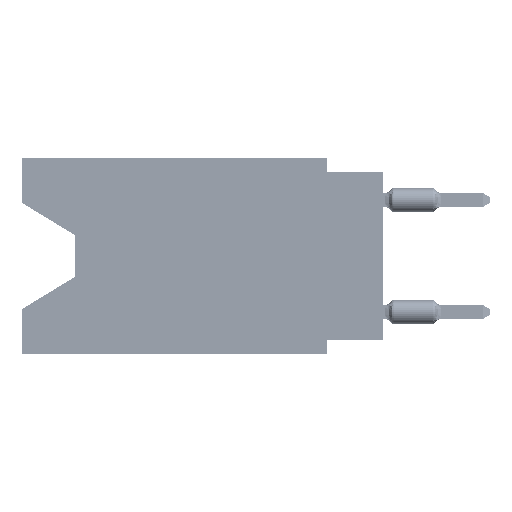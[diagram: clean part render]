
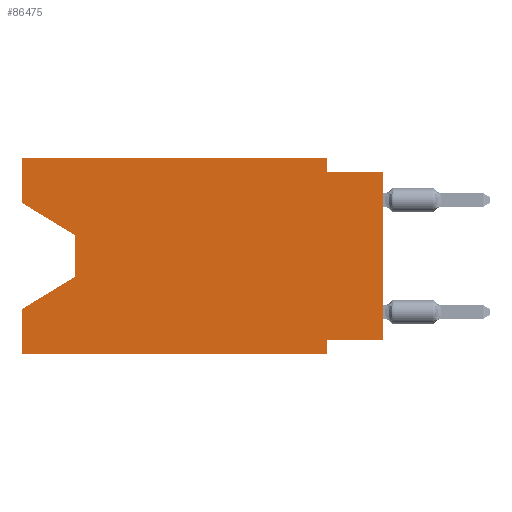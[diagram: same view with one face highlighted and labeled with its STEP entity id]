
A CAD part, left-side view. The second image highlights one B-rep face of the part: STEP entity #86475.
In plain terms, the highlighted planar face has unit normal (-1, 0, 0).
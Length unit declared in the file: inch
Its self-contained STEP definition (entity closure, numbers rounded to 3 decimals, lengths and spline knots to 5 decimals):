
#349 = VERTEX_POINT ( 'NONE', #7538 ) ;
#2107 = CARTESIAN_POINT ( 'NONE',  ( 0., 0.645, 0. ) ) ;
#2624 = CARTESIAN_POINT ( 'NONE',  ( 0., 0.645, -0.08025 ) ) ;
#6513 = VECTOR ( 'NONE', #92453, 39.37008 ) ;
#7045 = CARTESIAN_POINT ( 'NONE',  ( 0., 0.1, 0. ) ) ;
#7538 = CARTESIAN_POINT ( 'NONE',  ( 0., 0., -0.325 ) ) ;
#8836 = ORIENTED_EDGE ( 'NONE', *, *, #57607, .F. ) ;
#10146 = CARTESIAN_POINT ( 'NONE',  ( 0., 0.645, -0.08025 ) ) ;
#11338 = CARTESIAN_POINT ( 'NONE',  ( 0., 0.1, -0.325 ) ) ;
#13796 = VECTOR ( 'NONE', #97462, 39.37008 ) ;
#14514 = EDGE_CURVE ( 'NONE', #349, #19084, #79077, .T. ) ;
#14890 = CARTESIAN_POINT ( 'NONE',  ( 0., 0., -0.325 ) ) ;
#14999 = ORIENTED_EDGE ( 'NONE', *, *, #114864, .F. ) ;
#15421 = CARTESIAN_POINT ( 'NONE',  ( 0., 0., -0.025 ) ) ;
#15929 = VERTEX_POINT ( 'NONE', #10146 ) ;
#16733 = VECTOR ( 'NONE', #24178, 39.37008 ) ;
#17035 = CARTESIAN_POINT ( 'NONE',  ( 0., 0.645, -0.26975 ) ) ;
#19059 = VERTEX_POINT ( 'NONE', #98266 ) ;
#19084 = VERTEX_POINT ( 'NONE', #15421 ) ;
#20007 = CARTESIAN_POINT ( 'NONE',  ( 0., 0.645, -0.35 ) ) ;
#20026 = CARTESIAN_POINT ( 'NONE',  ( 0., 0.645, 0. ) ) ;
#20133 = DIRECTION ( 'NONE',  ( 1., 0., 0. ) ) ;
#20816 = CARTESIAN_POINT ( 'NONE',  ( 0., 0.645, -0.35 ) ) ;
#21044 = DIRECTION ( 'NONE',  ( 0., 0., -1. ) ) ;
#21537 = VECTOR ( 'NONE', #21627, 39.37008 ) ;
#21627 = DIRECTION ( 'NONE',  ( 0., 0., 1. ) ) ;
#24178 = DIRECTION ( 'NONE',  ( 0., 0., -1. ) ) ;
#25944 = LINE ( 'NONE', #106408, #16733 ) ;
#28666 = ORIENTED_EDGE ( 'NONE', *, *, #44477, .F. ) ;
#29025 = LINE ( 'NONE', #20026, #48783 ) ;
#29720 = FACE_OUTER_BOUND ( 'NONE', #41743, .T. ) ;
#33376 = LINE ( 'NONE', #98780, #70916 ) ;
#33512 = DIRECTION ( 'NONE',  ( 0., 1., 0. ) ) ;
#36156 = VERTEX_POINT ( 'NONE', #102610 ) ;
#36234 = LINE ( 'NONE', #20007, #63075 ) ;
#37456 = DIRECTION ( 'NONE',  ( 0., 0., 1. ) ) ;
#41038 = EDGE_CURVE ( 'NONE', #36156, #118572, #101459, .T. ) ;
#41161 = CARTESIAN_POINT ( 'NONE',  ( 0., 0.1, 0. ) ) ;
#41743 = EDGE_LOOP ( 'NONE', ( #59930, #54514, #58443, #102356, #45759, #75105, #109483, #89436, #8836, #14999, #93453, #28666 ) ) ;
#42187 = VERTEX_POINT ( 'NONE', #70476 ) ;
#44477 = EDGE_CURVE ( 'NONE', #15929, #50936, #100841, .T. ) ;
#44988 = VERTEX_POINT ( 'NONE', #20816 ) ;
#45626 = CARTESIAN_POINT ( 'NONE',  ( 0., 0.645, 0. ) ) ;
#45759 = ORIENTED_EDGE ( 'NONE', *, *, #81776, .T. ) ;
#47244 = CARTESIAN_POINT ( 'NONE',  ( 0., 0.1, -0.35 ) ) ;
#48263 = LINE ( 'NONE', #2624, #50380 ) ;
#48783 = VECTOR ( 'NONE', #37456, 39.37008 ) ;
#50380 = VECTOR ( 'NONE', #73653, 39.37008 ) ;
#50528 = EDGE_CURVE ( 'NONE', #50936, #108340, #63550, .T. ) ;
#50920 = LINE ( 'NONE', #14890, #78398 ) ;
#50936 = VERTEX_POINT ( 'NONE', #88046 ) ;
#54514 = ORIENTED_EDGE ( 'NONE', *, *, #100663, .T. ) ;
#55829 = CARTESIAN_POINT ( 'NONE',  ( 0., 0.55, -0.212 ) ) ;
#57446 = VERTEX_POINT ( 'NONE', #47244 ) ;
#57607 = EDGE_CURVE ( 'NONE', #19059, #19084, #33376, .T. ) ;
#58443 = ORIENTED_EDGE ( 'NONE', *, *, #41038, .T. ) ;
#59930 = ORIENTED_EDGE ( 'NONE', *, *, #109920, .T. ) ;
#63075 = VECTOR ( 'NONE', #99875, 39.37008 ) ;
#63176 = AXIS2_PLACEMENT_3D ( 'NONE', #2107, #20133, #112563 ) ;
#63550 = LINE ( 'NONE', #108000, #95547 ) ;
#64316 = EDGE_CURVE ( 'NONE', #44988, #118572, #29025, .T. ) ;
#67495 = LINE ( 'NONE', #69864, #13796 ) ;
#69292 = VERTEX_POINT ( 'NONE', #11338 ) ;
#69864 = CARTESIAN_POINT ( 'NONE',  ( 0., 0.1, -0.35 ) ) ;
#70476 = CARTESIAN_POINT ( 'NONE',  ( 0., 0.55, -0.138 ) ) ;
#70916 = VECTOR ( 'NONE', #116786, 39.37008 ) ;
#73653 = DIRECTION ( 'NONE',  ( 0., -0.855, -0.519 ) ) ;
#73721 = VECTOR ( 'NONE', #109864, 39.37008 ) ;
#75105 = ORIENTED_EDGE ( 'NONE', *, *, #107495, .F. ) ;
#75646 = CARTESIAN_POINT ( 'NONE',  ( 0., 0., 0. ) ) ;
#75916 = PLANE ( 'NONE',  #63176 ) ;
#78398 = VECTOR ( 'NONE', #33512, 39.37008 ) ;
#79077 = LINE ( 'NONE', #75646, #21537 ) ;
#81776 = EDGE_CURVE ( 'NONE', #44988, #57446, #36234, .T. ) ;
#86475 = ADVANCED_FACE ( 'NONE', ( #29720 ), #75916, .F. ) ;
#88046 = CARTESIAN_POINT ( 'NONE',  ( 0., 0.645, 0. ) ) ;
#89436 = ORIENTED_EDGE ( 'NONE', *, *, #14514, .T. ) ;
#92453 = DIRECTION ( 'NONE',  ( 0., 0.855, -0.519 ) ) ;
#93453 = ORIENTED_EDGE ( 'NONE', *, *, #50528, .F. ) ;
#95547 = VECTOR ( 'NONE', #110370, 39.37008 ) ;
#97133 = VECTOR ( 'NONE', #21044, 39.37008 ) ;
#97462 = DIRECTION ( 'NONE',  ( 0., 0., -1. ) ) ;
#98266 = CARTESIAN_POINT ( 'NONE',  ( 0., 0.1, -0.025 ) ) ;
#98780 = CARTESIAN_POINT ( 'NONE',  ( 0., 0., -0.025 ) ) ;
#99875 = DIRECTION ( 'NONE',  ( 0., -1., 0. ) ) ;
#100663 = EDGE_CURVE ( 'NONE', #42187, #36156, #25944, .T. ) ;
#100841 = LINE ( 'NONE', #45626, #73721 ) ;
#101459 = LINE ( 'NONE', #55829, #6513 ) ;
#102118 = LINE ( 'NONE', #7045, #97133 ) ;
#102356 = ORIENTED_EDGE ( 'NONE', *, *, #64316, .F. ) ;
#102610 = CARTESIAN_POINT ( 'NONE',  ( 0., 0.55, -0.212 ) ) ;
#104239 = EDGE_CURVE ( 'NONE', #349, #69292, #50920, .T. ) ;
#106408 = CARTESIAN_POINT ( 'NONE',  ( 0., 0.55, -0.138 ) ) ;
#107495 = EDGE_CURVE ( 'NONE', #69292, #57446, #67495, .T. ) ;
#108000 = CARTESIAN_POINT ( 'NONE',  ( 0., 0.645, 0. ) ) ;
#108340 = VERTEX_POINT ( 'NONE', #41161 ) ;
#109483 = ORIENTED_EDGE ( 'NONE', *, *, #104239, .F. ) ;
#109864 = DIRECTION ( 'NONE',  ( 0., 0., 1. ) ) ;
#109920 = EDGE_CURVE ( 'NONE', #15929, #42187, #48263, .T. ) ;
#110370 = DIRECTION ( 'NONE',  ( 0., -1., 0. ) ) ;
#112563 = DIRECTION ( 'NONE',  ( 0., 0., -1. ) ) ;
#114864 = EDGE_CURVE ( 'NONE', #108340, #19059, #102118, .T. ) ;
#116786 = DIRECTION ( 'NONE',  ( 0., -1., 0. ) ) ;
#118572 = VERTEX_POINT ( 'NONE', #17035 ) ;
